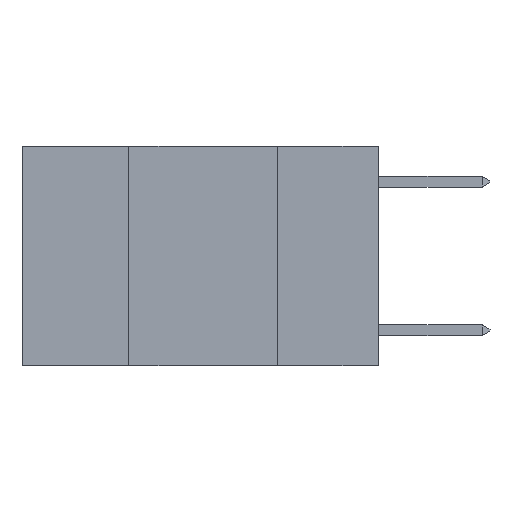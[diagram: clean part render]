
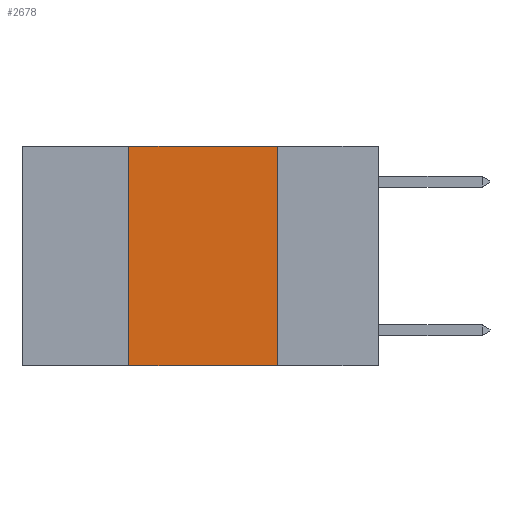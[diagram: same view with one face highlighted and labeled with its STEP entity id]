
A CAD part, left-side view. The second image highlights one B-rep face of the part: STEP entity #2678.
In plain terms, the highlighted planar face has unit normal (-1, 0, 0).
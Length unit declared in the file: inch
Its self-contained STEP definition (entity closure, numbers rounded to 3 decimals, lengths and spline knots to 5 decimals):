
#1532 = DIRECTION ( 'NONE',  ( 0., 0., -1. ) ) ;
#1900 = DIRECTION ( 'NONE',  ( 0., -1., 0. ) ) ;
#2326 = CARTESIAN_POINT ( 'NONE',  ( 0., 0.42, 0. ) ) ;
#2483 = EDGE_LOOP ( 'NONE', ( #15252, #14988, #15492, #8828 ) ) ;
#2678 = ADVANCED_FACE ( 'NONE', ( #5888 ), #6417, .F. ) ;
#2935 = AXIS2_PLACEMENT_3D ( 'NONE', #6597, #6191, #5962 ) ;
#2975 = DIRECTION ( 'NONE',  ( 0., -1., 0. ) ) ;
#3382 = LINE ( 'NONE', #5803, #10500 ) ;
#4975 = LINE ( 'NONE', #14619, #12468 ) ;
#4982 = EDGE_CURVE ( 'NONE', #7896, #9760, #3382, .T. ) ;
#5800 = CARTESIAN_POINT ( 'NONE',  ( 0., 0.6, -0.37 ) ) ;
#5803 = CARTESIAN_POINT ( 'NONE',  ( 0., 0.17, 0. ) ) ;
#5888 = FACE_OUTER_BOUND ( 'NONE', #2483, .T. ) ;
#5962 = DIRECTION ( 'NONE',  ( 0., 0., -1. ) ) ;
#6191 = DIRECTION ( 'NONE',  ( 1., 0., 0. ) ) ;
#6417 = PLANE ( 'NONE',  #2935 ) ;
#6465 = CARTESIAN_POINT ( 'NONE',  ( 0., 0.17, 0. ) ) ;
#6597 = CARTESIAN_POINT ( 'NONE',  ( 0., 0.6, 0. ) ) ;
#7410 = LINE ( 'NONE', #2326, #17810 ) ;
#7511 = LINE ( 'NONE', #5800, #14074 ) ;
#7896 = VERTEX_POINT ( 'NONE', #6465 ) ;
#8828 = ORIENTED_EDGE ( 'NONE', *, *, #14730, .T. ) ;
#9120 = CARTESIAN_POINT ( 'NONE',  ( 0., 0.17, -0.37 ) ) ;
#9760 = VERTEX_POINT ( 'NONE', #9120 ) ;
#10500 = VECTOR ( 'NONE', #1532, 39.37008 ) ;
#10591 = VERTEX_POINT ( 'NONE', #12194 ) ;
#12194 = CARTESIAN_POINT ( 'NONE',  ( 0., 0.42, -0.37 ) ) ;
#12468 = VECTOR ( 'NONE', #1900, 39.37008 ) ;
#12558 = CARTESIAN_POINT ( 'NONE',  ( 0., 0.42, 0. ) ) ;
#13706 = DIRECTION ( 'NONE',  ( 0., 0., 1. ) ) ;
#14074 = VECTOR ( 'NONE', #2975, 39.37008 ) ;
#14619 = CARTESIAN_POINT ( 'NONE',  ( 0., 0.6, 0. ) ) ;
#14730 = EDGE_CURVE ( 'NONE', #10591, #9760, #7511, .T. ) ;
#14988 = ORIENTED_EDGE ( 'NONE', *, *, #17392, .F. ) ;
#15252 = ORIENTED_EDGE ( 'NONE', *, *, #4982, .F. ) ;
#15271 = VERTEX_POINT ( 'NONE', #12558 ) ;
#15492 = ORIENTED_EDGE ( 'NONE', *, *, #16446, .F. ) ;
#16446 = EDGE_CURVE ( 'NONE', #10591, #15271, #7410, .T. ) ;
#17392 = EDGE_CURVE ( 'NONE', #15271, #7896, #4975, .T. ) ;
#17810 = VECTOR ( 'NONE', #13706, 39.37008 ) ;
